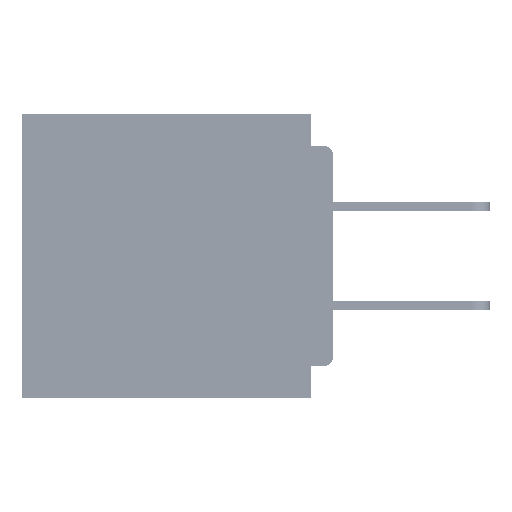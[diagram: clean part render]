
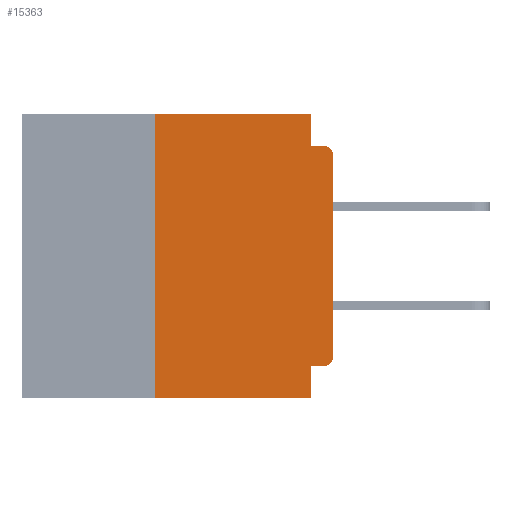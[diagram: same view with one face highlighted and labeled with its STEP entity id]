
A CAD part, left-side view. The second image highlights one B-rep face of the part: STEP entity #15363.
In plain terms, the highlighted planar face has unit normal (-1, 0, 0).
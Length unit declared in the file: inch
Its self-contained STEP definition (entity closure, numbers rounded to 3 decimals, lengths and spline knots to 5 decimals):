
#436 = VECTOR ( 'NONE', #24519, 39.37008 ) ;
#567 = VECTOR ( 'NONE', #5545, 39.37008 ) ;
#580 = CARTESIAN_POINT ( 'NONE',  ( 0., 0., -0.045 ) ) ;
#744 = CARTESIAN_POINT ( 'NONE',  ( 0., 0., -0.34 ) ) ;
#1756 = VERTEX_POINT ( 'NONE', #57039 ) ;
#2450 = CARTESIAN_POINT ( 'NONE',  ( 0., 0.25, -0.4 ) ) ;
#2876 = DIRECTION ( 'NONE',  ( 1., 0., 0. ) ) ;
#3364 = DIRECTION ( 'NONE',  ( 0., 0., 1. ) ) ;
#3936 = ORIENTED_EDGE ( 'NONE', *, *, #22298, .F. ) ;
#5221 = LINE ( 'NONE', #60910, #43181 ) ;
#5545 = DIRECTION ( 'NONE',  ( 0., -1., 0. ) ) ;
#5746 = VERTEX_POINT ( 'NONE', #50411 ) ;
#6032 = DIRECTION ( 'NONE',  ( -1., 0., 0. ) ) ;
#7665 = CARTESIAN_POINT ( 'NONE',  ( 0., 0.437, 0. ) ) ;
#8878 = ORIENTED_EDGE ( 'NONE', *, *, #36554, .F. ) ;
#9718 = VERTEX_POINT ( 'NONE', #13701 ) ;
#11175 = DIRECTION ( 'NONE',  ( 0., 0., 1. ) ) ;
#11304 = LINE ( 'NONE', #45814, #22868 ) ;
#11705 = ORIENTED_EDGE ( 'NONE', *, *, #30056, .F. ) ;
#13060 = EDGE_CURVE ( 'NONE', #60246, #47362, #5221, .T. ) ;
#13701 = CARTESIAN_POINT ( 'NONE',  ( 0., 0.031, -0.045 ) ) ;
#15363 = ADVANCED_FACE ( 'NONE', ( #36652 ), #57080, .F. ) ;
#16455 = DIRECTION ( 'NONE',  ( 0., -1., 0. ) ) ;
#16868 = VECTOR ( 'NONE', #61569, 39.37008 ) ;
#17453 = ORIENTED_EDGE ( 'NONE', *, *, #30720, .F. ) ;
#18731 = CARTESIAN_POINT ( 'NONE',  ( 0., 0.031, 0. ) ) ;
#22298 = EDGE_CURVE ( 'NONE', #63314, #47362, #53197, .T. ) ;
#22868 = VECTOR ( 'NONE', #11175, 39.37008 ) ;
#24519 = DIRECTION ( 'NONE',  ( 0., 0., -1. ) ) ;
#24743 = CARTESIAN_POINT ( 'NONE',  ( 0., 0.25, 0. ) ) ;
#25634 = EDGE_LOOP ( 'NONE', ( #36993, #36981, #42311, #17453, #40537, #11705, #33236, #3936, #8878, #50934 ) ) ;
#26815 = VERTEX_POINT ( 'NONE', #24743 ) ;
#27276 = DIRECTION ( 'NONE',  ( 0., 0., -1. ) ) ;
#29347 = DIRECTION ( 'NONE',  ( -1., 0., 0. ) ) ;
#30056 = EDGE_CURVE ( 'NONE', #60246, #26815, #11304, .T. ) ;
#30720 = EDGE_CURVE ( 'NONE', #33944, #9718, #60061, .T. ) ;
#31825 = VERTEX_POINT ( 'NONE', #52112 ) ;
#33072 = CIRCLE ( 'NONE', #60434, 0.015 ) ;
#33197 = EDGE_CURVE ( 'NONE', #33504, #31825, #41933, .T. ) ;
#33236 = ORIENTED_EDGE ( 'NONE', *, *, #13060, .T. ) ;
#33504 = VERTEX_POINT ( 'NONE', #744 ) ;
#33944 = VERTEX_POINT ( 'NONE', #18731 ) ;
#35173 = VECTOR ( 'NONE', #27276, 39.37008 ) ;
#35657 = CARTESIAN_POINT ( 'NONE',  ( 0., 0.015, -0.34 ) ) ;
#36554 = EDGE_CURVE ( 'NONE', #1756, #63314, #56382, .T. ) ;
#36652 = FACE_OUTER_BOUND ( 'NONE', #25634, .T. ) ;
#36913 = CARTESIAN_POINT ( 'NONE',  ( 0., 0.031, -0.355 ) ) ;
#36981 = ORIENTED_EDGE ( 'NONE', *, *, #62951, .T. ) ;
#36993 = ORIENTED_EDGE ( 'NONE', *, *, #33197, .T. ) ;
#37523 = DIRECTION ( 'NONE',  ( 0., 0., -1. ) ) ;
#38821 = CIRCLE ( 'NONE', #55156, 0.015 ) ;
#40380 = VECTOR ( 'NONE', #3364, 39.37008 ) ;
#40537 = ORIENTED_EDGE ( 'NONE', *, *, #43738, .F. ) ;
#40691 = DIRECTION ( 'NONE',  ( 0., 0., -1. ) ) ;
#41933 = LINE ( 'NONE', #52821, #40380 ) ;
#42311 = ORIENTED_EDGE ( 'NONE', *, *, #63069, .F. ) ;
#42709 = CARTESIAN_POINT ( 'NONE',  ( 0., 0.031, -0.4 ) ) ;
#43181 = VECTOR ( 'NONE', #16455, 39.37008 ) ;
#43738 = EDGE_CURVE ( 'NONE', #26815, #33944, #56447, .T. ) ;
#43788 = CARTESIAN_POINT ( 'NONE',  ( 0., 0., -0.355 ) ) ;
#43941 = AXIS2_PLACEMENT_3D ( 'NONE', #7665, #2876, #37523 ) ;
#45814 = CARTESIAN_POINT ( 'NONE',  ( 0., 0.25, -0.4 ) ) ;
#47038 = CARTESIAN_POINT ( 'NONE',  ( 0., 0.031, 0. ) ) ;
#47362 = VERTEX_POINT ( 'NONE', #42709 ) ;
#50411 = CARTESIAN_POINT ( 'NONE',  ( 0., 0.015, -0.045 ) ) ;
#50934 = ORIENTED_EDGE ( 'NONE', *, *, #55022, .T. ) ;
#51613 = CARTESIAN_POINT ( 'NONE',  ( 0., 0.437, 0. ) ) ;
#52112 = CARTESIAN_POINT ( 'NONE',  ( 0., 0., -0.06 ) ) ;
#52821 = CARTESIAN_POINT ( 'NONE',  ( 0., 0., 0. ) ) ;
#53197 = LINE ( 'NONE', #59258, #436 ) ;
#53287 = VECTOR ( 'NONE', #63727, 39.37008 ) ;
#54885 = LINE ( 'NONE', #580, #567 ) ;
#55022 = EDGE_CURVE ( 'NONE', #1756, #33504, #38821, .T. ) ;
#55156 = AXIS2_PLACEMENT_3D ( 'NONE', #35657, #6032, #40691 ) ;
#56382 = LINE ( 'NONE', #43788, #53287 ) ;
#56447 = LINE ( 'NONE', #51613, #16868 ) ;
#57039 = CARTESIAN_POINT ( 'NONE',  ( 0., 0.015, -0.355 ) ) ;
#57080 = PLANE ( 'NONE',  #43941 ) ;
#59097 = CARTESIAN_POINT ( 'NONE',  ( 0., 0.015, -0.06 ) ) ;
#59258 = CARTESIAN_POINT ( 'NONE',  ( 0., 0.031, -0.4 ) ) ;
#60061 = LINE ( 'NONE', #47038, #35173 ) ;
#60246 = VERTEX_POINT ( 'NONE', #2450 ) ;
#60434 = AXIS2_PLACEMENT_3D ( 'NONE', #59097, #29347, #64042 ) ;
#60910 = CARTESIAN_POINT ( 'NONE',  ( 0., 0.437, -0.4 ) ) ;
#61569 = DIRECTION ( 'NONE',  ( 0., -1., 0. ) ) ;
#62951 = EDGE_CURVE ( 'NONE', #31825, #5746, #33072, .T. ) ;
#63069 = EDGE_CURVE ( 'NONE', #9718, #5746, #54885, .T. ) ;
#63314 = VERTEX_POINT ( 'NONE', #36913 ) ;
#63727 = DIRECTION ( 'NONE',  ( 0., 1., 0. ) ) ;
#64042 = DIRECTION ( 'NONE',  ( 0., 0., -1. ) ) ;
